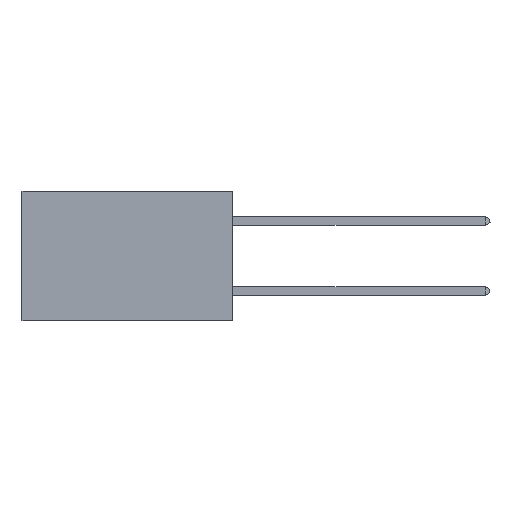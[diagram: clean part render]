
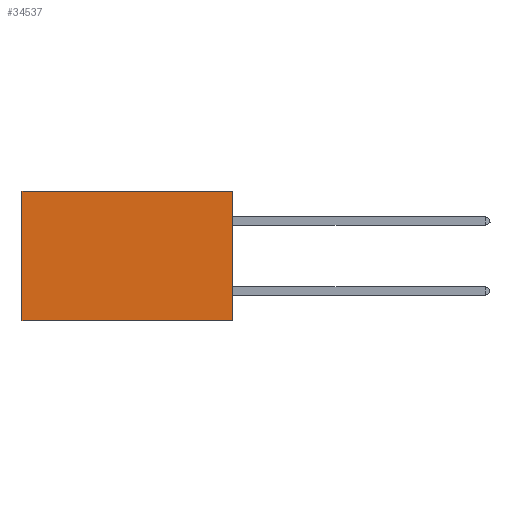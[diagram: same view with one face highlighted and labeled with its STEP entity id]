
A CAD part, left-side view. The second image highlights one B-rep face of the part: STEP entity #34537.
In plain terms, the highlighted planar face has unit normal (-1, 0, 0).
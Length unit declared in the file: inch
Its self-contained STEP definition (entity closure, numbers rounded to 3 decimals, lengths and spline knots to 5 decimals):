
#293 = EDGE_CURVE ( 'NONE', #34056, #351, #30490, .T. ) ;
#351 = VERTEX_POINT ( 'NONE', #33537 ) ;
#2438 = VECTOR ( 'NONE', #4485, 39.37008 ) ;
#4485 = DIRECTION ( 'NONE',  ( 0., 0., -1. ) ) ;
#4766 = EDGE_CURVE ( 'NONE', #37770, #351, #12384, .T. ) ;
#6921 = ORIENTED_EDGE ( 'NONE', *, *, #4766, .T. ) ;
#7000 = DIRECTION ( 'NONE',  ( 0., 0., -1. ) ) ;
#7841 = DIRECTION ( 'NONE',  ( 0., 0., -1. ) ) ;
#9702 = VECTOR ( 'NONE', #7000, 39.37008 ) ;
#12384 = LINE ( 'NONE', #22962, #2438 ) ;
#16500 = ORIENTED_EDGE ( 'NONE', *, *, #31461, .T. ) ;
#17796 = VECTOR ( 'NONE', #43537, 39.37008 ) ;
#18095 = CARTESIAN_POINT ( 'NONE',  ( 0.2875, 0., 0. ) ) ;
#19398 = DIRECTION ( 'NONE',  ( 0., 1., 0. ) ) ;
#19480 = LINE ( 'NONE', #25379, #9702 ) ;
#19799 = ORIENTED_EDGE ( 'NONE', *, *, #21240, .F. ) ;
#21240 = EDGE_CURVE ( 'NONE', #21676, #34056, #19480, .T. ) ;
#21676 = VERTEX_POINT ( 'NONE', #42659 ) ;
#22499 = CARTESIAN_POINT ( 'NONE',  ( 0.2875, 0., 0. ) ) ;
#22962 = CARTESIAN_POINT ( 'NONE',  ( 0.2875, 0.6, 0. ) ) ;
#25379 = CARTESIAN_POINT ( 'NONE',  ( 0.2875, 0., 0. ) ) ;
#27458 = CARTESIAN_POINT ( 'NONE',  ( 0.2875, 0., -0.37 ) ) ;
#28261 = CARTESIAN_POINT ( 'NONE',  ( 0.2875, 0.6, 0. ) ) ;
#29347 = VECTOR ( 'NONE', #19398, 39.37008 ) ;
#29813 = DIRECTION ( 'NONE',  ( 1., 0., 0. ) ) ;
#30490 = LINE ( 'NONE', #37943, #29347 ) ;
#31461 = EDGE_CURVE ( 'NONE', #21676, #37770, #45646, .T. ) ;
#33537 = CARTESIAN_POINT ( 'NONE',  ( 0.2875, 0.6, -0.37 ) ) ;
#34056 = VERTEX_POINT ( 'NONE', #27458 ) ;
#34537 = ADVANCED_FACE ( 'NONE', ( #38002 ), #44251, .F. ) ;
#35534 = ORIENTED_EDGE ( 'NONE', *, *, #293, .F. ) ;
#37770 = VERTEX_POINT ( 'NONE', #28261 ) ;
#37943 = CARTESIAN_POINT ( 'NONE',  ( 0.2875, 0., -0.37 ) ) ;
#38002 = FACE_OUTER_BOUND ( 'NONE', #47438, .T. ) ;
#38547 = AXIS2_PLACEMENT_3D ( 'NONE', #22499, #29813, #7841 ) ;
#42659 = CARTESIAN_POINT ( 'NONE',  ( 0.2875, 0., 0. ) ) ;
#43537 = DIRECTION ( 'NONE',  ( 0., 1., 0. ) ) ;
#44251 = PLANE ( 'NONE',  #38547 ) ;
#45646 = LINE ( 'NONE', #18095, #17796 ) ;
#47438 = EDGE_LOOP ( 'NONE', ( #6921, #35534, #19799, #16500 ) ) ;
